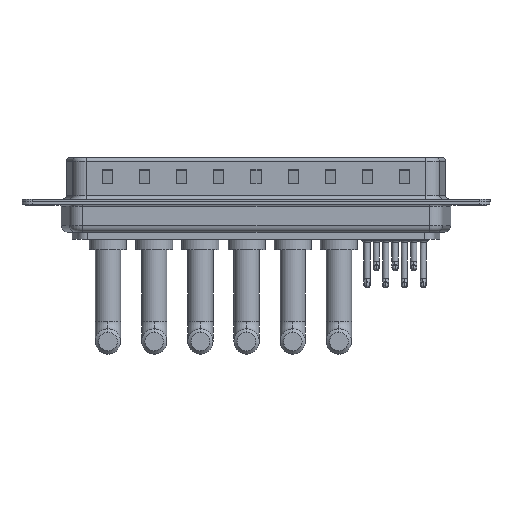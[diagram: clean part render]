
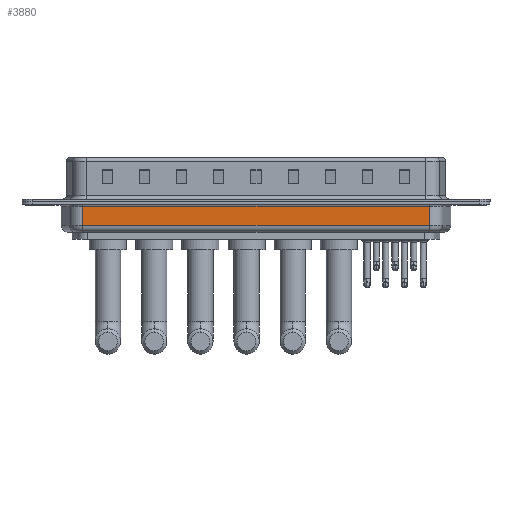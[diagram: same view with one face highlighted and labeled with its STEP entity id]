
A CAD part, front view. The second image highlights one B-rep face of the part: STEP entity #3880.
In plain terms, the highlighted planar face has unit normal (0, -1, 0).
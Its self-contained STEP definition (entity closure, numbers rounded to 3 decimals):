
#244 = FACE_OUTER_BOUND ( 'NONE', #15436, .T. ) ;
#442 = DIRECTION ( 'NONE',  ( -1., 0., 0. ) ) ;
#1152 = CARTESIAN_POINT ( 'NONE',  ( 57.469, -5.35, -0.65 ) ) ;
#2130 = ORIENTED_EDGE ( 'NONE', *, *, #6637, .T. ) ;
#2518 = VECTOR ( 'NONE', #16942, 1000. ) ;
#2696 = VECTOR ( 'NONE', #15831, 1000. ) ;
#3235 = CARTESIAN_POINT ( 'NONE',  ( 6.031, -5.35, -4.5 ) ) ;
#3880 = ADVANCED_FACE ( 'NONE', ( #244 ), #22507, .F. ) ;
#5027 = ORIENTED_EDGE ( 'NONE', *, *, #21090, .F. ) ;
#5083 = CARTESIAN_POINT ( 'NONE',  ( 6.031, -5.35, -4.5 ) ) ;
#5336 = VERTEX_POINT ( 'NONE', #20542 ) ;
#5602 = LINE ( 'NONE', #14213, #17459 ) ;
#5685 = VERTEX_POINT ( 'NONE', #1152 ) ;
#6374 = AXIS2_PLACEMENT_3D ( 'NONE', #3235, #21109, #6772 ) ;
#6637 = EDGE_CURVE ( 'NONE', #5336, #16605, #22396, .T. ) ;
#6661 = CARTESIAN_POINT ( 'NONE',  ( 6.031, -5.35, -3.5 ) ) ;
#6772 = DIRECTION ( 'NONE',  ( -1., 0., 0. ) ) ;
#8856 = DIRECTION ( 'NONE',  ( 0., 0., 1. ) ) ;
#10291 = CARTESIAN_POINT ( 'NONE',  ( 57.469, -5.35, -4.5 ) ) ;
#10342 = LINE ( 'NONE', #5083, #14856 ) ;
#11783 = EDGE_CURVE ( 'NONE', #5685, #14230, #5602, .T. ) ;
#12751 = ORIENTED_EDGE ( 'NONE', *, *, #14263, .T. ) ;
#12858 = ORIENTED_EDGE ( 'NONE', *, *, #11783, .T. ) ;
#14213 = CARTESIAN_POINT ( 'NONE',  ( 6.031, -5.35, -0.65 ) ) ;
#14230 = VERTEX_POINT ( 'NONE', #18556 ) ;
#14263 = EDGE_CURVE ( 'NONE', #16605, #5685, #19008, .T. ) ;
#14367 = CARTESIAN_POINT ( 'NONE',  ( 57.469, -5.35, -3.5 ) ) ;
#14856 = VECTOR ( 'NONE', #8856, 1000. ) ;
#15436 = EDGE_LOOP ( 'NONE', ( #5027, #2130, #12751, #12858 ) ) ;
#15831 = DIRECTION ( 'NONE',  ( 1., 0., 0. ) ) ;
#16605 = VERTEX_POINT ( 'NONE', #14367 ) ;
#16942 = DIRECTION ( 'NONE',  ( 0., 0., 1. ) ) ;
#17459 = VECTOR ( 'NONE', #442, 1000. ) ;
#18556 = CARTESIAN_POINT ( 'NONE',  ( 6.031, -5.35, -0.65 ) ) ;
#19008 = LINE ( 'NONE', #10291, #2518 ) ;
#20542 = CARTESIAN_POINT ( 'NONE',  ( 6.031, -5.35, -3.5 ) ) ;
#21090 = EDGE_CURVE ( 'NONE', #5336, #14230, #10342, .T. ) ;
#21109 = DIRECTION ( 'NONE',  ( 0., 1., 0. ) ) ;
#22396 = LINE ( 'NONE', #6661, #2696 ) ;
#22507 = PLANE ( 'NONE',  #6374 ) ;
